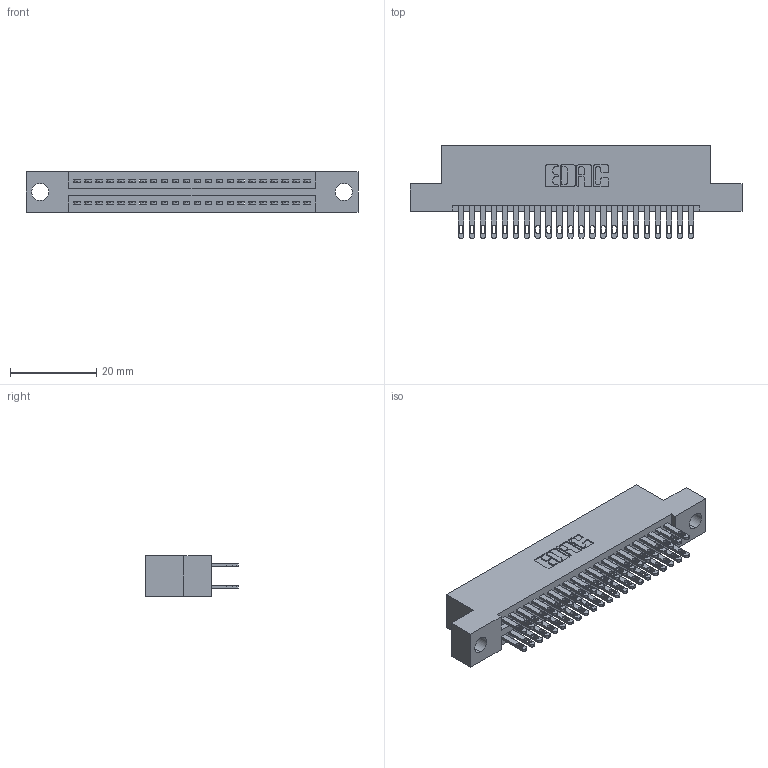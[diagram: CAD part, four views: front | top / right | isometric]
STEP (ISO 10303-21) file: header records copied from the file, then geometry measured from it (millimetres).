
FILE_DESCRIPTION (( 'STEP AP203' ), '1' );
FILE_NAME ('345-044-500-204.STEP', '2021-05-20T01:47:21', ( '' ), ( '' ), 'SwSTEP 2.0', 'SolidWorks 2020', '' );
FILE_SCHEMA (( 'CONFIG_CONTROL_DESIGN' ));
Length unit declared in the file: inch
Products named in the file (3): 345-044-500-204; 345 Part_Flush Mounting Lugs - 0.156 Dia-TI; 345-292-001_345-293-100
Assembly tree (45 placements, depth 2):
  345-044-500-204
    345 Part_Flush Mounting Lugs - 0.156 Dia-TI
    345-292-001_345-293-100  x44
Bounding box: 77.09 x 21.51 x 9.4 mm (x, y, z)
Volume: 7331.4 mm3; surface area: 10750 mm2
Topology: 45 solids, 45 shells, 2164 faces, 6581 edges, 4386 vertices
Faces by surface type: plane 1282, cylinder 882
Entity records: 20303 total; most frequent: CARTESIAN_POINT 3426, ORIENTED_EDGE 3358, DIRECTION 3047, EDGE_CURVE 1679, VECTOR 1455, LINE 1455, VERTEX_POINT 1118, AXIS2_PLACEMENT_3D 796
